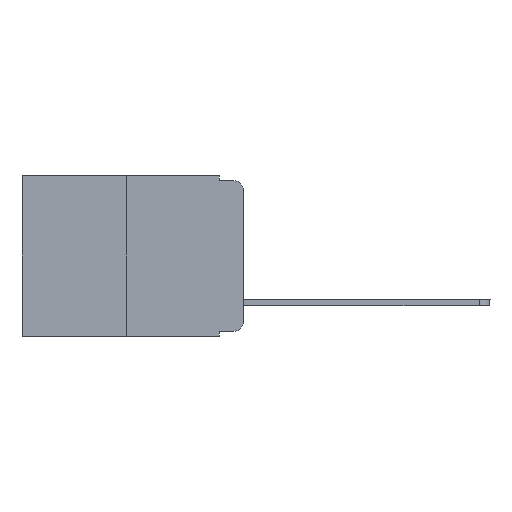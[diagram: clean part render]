
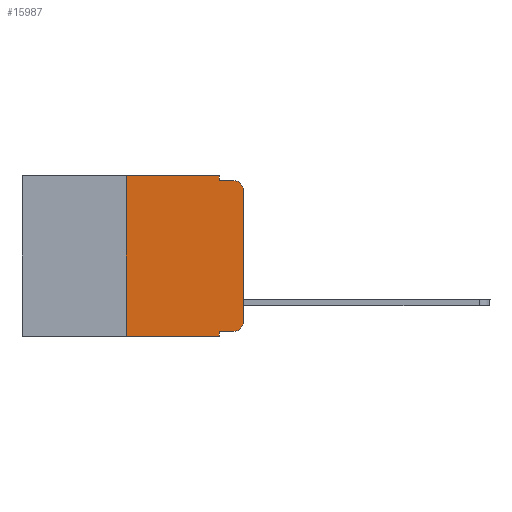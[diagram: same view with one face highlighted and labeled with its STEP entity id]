
A CAD part, left-side view. The second image highlights one B-rep face of the part: STEP entity #15987.
In plain terms, the highlighted planar face has unit normal (-1, 0, 0).
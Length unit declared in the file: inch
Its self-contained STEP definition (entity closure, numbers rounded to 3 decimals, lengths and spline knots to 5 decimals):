
#210 = DIRECTION ( 'NONE',  ( 0., -1., 0. ) ) ;
#329 = CARTESIAN_POINT ( 'NONE',  ( 0., 0.473, 0. ) ) ;
#709 = CARTESIAN_POINT ( 'NONE',  ( 0., 0.02, -0.313 ) ) ;
#853 = VECTOR ( 'NONE', #210, 39.37008 ) ;
#1753 = VECTOR ( 'NONE', #21927, 39.37008 ) ;
#1954 = LINE ( 'NONE', #21207, #10415 ) ;
#2063 = FACE_OUTER_BOUND ( 'NONE', #20187, .T. ) ;
#2198 = CARTESIAN_POINT ( 'NONE',  ( 0., 0.02, -0.333 ) ) ;
#2535 = DIRECTION ( 'NONE',  ( 0., 0., -1. ) ) ;
#2570 = EDGE_CURVE ( 'NONE', #20467, #22042, #10978, .T. ) ;
#3201 = LINE ( 'NONE', #12702, #6080 ) ;
#3761 = VERTEX_POINT ( 'NONE', #8826 ) ;
#4359 = VERTEX_POINT ( 'NONE', #17735 ) ;
#4386 = PLANE ( 'NONE',  #24922 ) ;
#4874 = VECTOR ( 'NONE', #15213, 39.37008 ) ;
#5884 = CARTESIAN_POINT ( 'NONE',  ( 0., 0.051, 0. ) ) ;
#6080 = VECTOR ( 'NONE', #15018, 39.37008 ) ;
#6265 = LINE ( 'NONE', #12045, #1753 ) ;
#6491 = VERTEX_POINT ( 'NONE', #23247 ) ;
#6881 = VERTEX_POINT ( 'NONE', #20449 ) ;
#7124 = DIRECTION ( 'NONE',  ( -1., 0., 0. ) ) ;
#7374 = CARTESIAN_POINT ( 'NONE',  ( 0., 0.02, -0.03 ) ) ;
#7985 = VECTOR ( 'NONE', #11923, 39.37008 ) ;
#8637 = CARTESIAN_POINT ( 'NONE',  ( 0., 0.02, -0.01 ) ) ;
#8826 = CARTESIAN_POINT ( 'NONE',  ( 0., 0., -0.313 ) ) ;
#10415 = VECTOR ( 'NONE', #19274, 39.37008 ) ;
#10464 = CARTESIAN_POINT ( 'NONE',  ( 0., 0.051, -0.333 ) ) ;
#10773 = EDGE_CURVE ( 'NONE', #21843, #25239, #6265, .T. ) ;
#10806 = EDGE_CURVE ( 'NONE', #16064, #3761, #19374, .T. ) ;
#10963 = DIRECTION ( 'NONE',  ( 0., 0., -1. ) ) ;
#10978 = LINE ( 'NONE', #24448, #4874 ) ;
#11488 = ORIENTED_EDGE ( 'NONE', *, *, #11516, .F. ) ;
#11516 = EDGE_CURVE ( 'NONE', #21843, #12875, #1954, .T. ) ;
#11923 = DIRECTION ( 'NONE',  ( 0., 0., -1. ) ) ;
#12045 = CARTESIAN_POINT ( 'NONE',  ( 0., 0.473, -0.343 ) ) ;
#12164 = LINE ( 'NONE', #329, #853 ) ;
#12191 = CARTESIAN_POINT ( 'NONE',  ( 0., 0.051, -0.01 ) ) ;
#12442 = CIRCLE ( 'NONE', #21455, 0.02 ) ;
#12467 = EDGE_CURVE ( 'NONE', #4359, #16064, #20076, .T. ) ;
#12635 = EDGE_CURVE ( 'NONE', #6491, #22042, #12442, .T. ) ;
#12702 = CARTESIAN_POINT ( 'NONE',  ( 0., 0., 0. ) ) ;
#12875 = VERTEX_POINT ( 'NONE', #23504 ) ;
#13278 = EDGE_CURVE ( 'NONE', #4359, #25239, #13457, .T. ) ;
#13457 = LINE ( 'NONE', #5884, #7985 ) ;
#13505 = CARTESIAN_POINT ( 'NONE',  ( 0., 0.051, 0. ) ) ;
#13774 = LINE ( 'NONE', #13505, #18795 ) ;
#14271 = DIRECTION ( 'NONE',  ( 0., 0., -1. ) ) ;
#14390 = CARTESIAN_POINT ( 'NONE',  ( 0., 0.473, 0. ) ) ;
#15018 = DIRECTION ( 'NONE',  ( 0., 0., 1. ) ) ;
#15213 = DIRECTION ( 'NONE',  ( 0., -1., 0. ) ) ;
#15978 = ORIENTED_EDGE ( 'NONE', *, *, #12635, .T. ) ;
#15987 = ADVANCED_FACE ( 'NONE', ( #2063 ), #4386, .F. ) ;
#16064 = VERTEX_POINT ( 'NONE', #2198 ) ;
#16991 = VECTOR ( 'NONE', #18391, 39.37008 ) ;
#17559 = EDGE_CURVE ( 'NONE', #3761, #6491, #3201, .T. ) ;
#17735 = CARTESIAN_POINT ( 'NONE',  ( 0., 0.051, -0.333 ) ) ;
#18206 = ORIENTED_EDGE ( 'NONE', *, *, #20865, .F. ) ;
#18391 = DIRECTION ( 'NONE',  ( 0., -1., 0. ) ) ;
#18593 = EDGE_CURVE ( 'NONE', #6881, #20467, #13774, .T. ) ;
#18795 = VECTOR ( 'NONE', #21321, 39.37008 ) ;
#19274 = DIRECTION ( 'NONE',  ( 0., 0., 1. ) ) ;
#19287 = CARTESIAN_POINT ( 'NONE',  ( 0., 0.25, -0.343 ) ) ;
#19374 = CIRCLE ( 'NONE', #21028, 0.02 ) ;
#19733 = ORIENTED_EDGE ( 'NONE', *, *, #10806, .T. ) ;
#19838 = ORIENTED_EDGE ( 'NONE', *, *, #18593, .F. ) ;
#20076 = LINE ( 'NONE', #10464, #16991 ) ;
#20187 = EDGE_LOOP ( 'NONE', ( #24485, #15978, #23629, #19838, #18206, #11488, #21618, #20950, #20825, #19733 ) ) ;
#20449 = CARTESIAN_POINT ( 'NONE',  ( 0., 0.051, 0. ) ) ;
#20467 = VERTEX_POINT ( 'NONE', #12191 ) ;
#20825 = ORIENTED_EDGE ( 'NONE', *, *, #12467, .T. ) ;
#20865 = EDGE_CURVE ( 'NONE', #12875, #6881, #12164, .T. ) ;
#20950 = ORIENTED_EDGE ( 'NONE', *, *, #13278, .F. ) ;
#21028 = AXIS2_PLACEMENT_3D ( 'NONE', #709, #22046, #2535 ) ;
#21047 = CARTESIAN_POINT ( 'NONE',  ( 0., 0.051, -0.343 ) ) ;
#21207 = CARTESIAN_POINT ( 'NONE',  ( 0., 0.25, 0. ) ) ;
#21321 = DIRECTION ( 'NONE',  ( 0., 0., -1. ) ) ;
#21455 = AXIS2_PLACEMENT_3D ( 'NONE', #7374, #7124, #10963 ) ;
#21618 = ORIENTED_EDGE ( 'NONE', *, *, #10773, .T. ) ;
#21843 = VERTEX_POINT ( 'NONE', #19287 ) ;
#21927 = DIRECTION ( 'NONE',  ( 0., -1., 0. ) ) ;
#22042 = VERTEX_POINT ( 'NONE', #8637 ) ;
#22046 = DIRECTION ( 'NONE',  ( -1., 0., 0. ) ) ;
#22209 = DIRECTION ( 'NONE',  ( 1., 0., 0. ) ) ;
#23247 = CARTESIAN_POINT ( 'NONE',  ( 0., 0., -0.03 ) ) ;
#23504 = CARTESIAN_POINT ( 'NONE',  ( 0., 0.25, 0. ) ) ;
#23629 = ORIENTED_EDGE ( 'NONE', *, *, #2570, .F. ) ;
#24448 = CARTESIAN_POINT ( 'NONE',  ( 0., 0.051, -0.01 ) ) ;
#24485 = ORIENTED_EDGE ( 'NONE', *, *, #17559, .T. ) ;
#24922 = AXIS2_PLACEMENT_3D ( 'NONE', #14390, #22209, #14271 ) ;
#25239 = VERTEX_POINT ( 'NONE', #21047 ) ;
